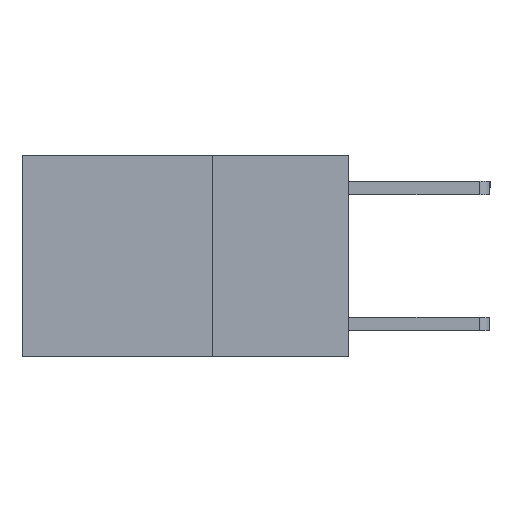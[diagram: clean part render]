
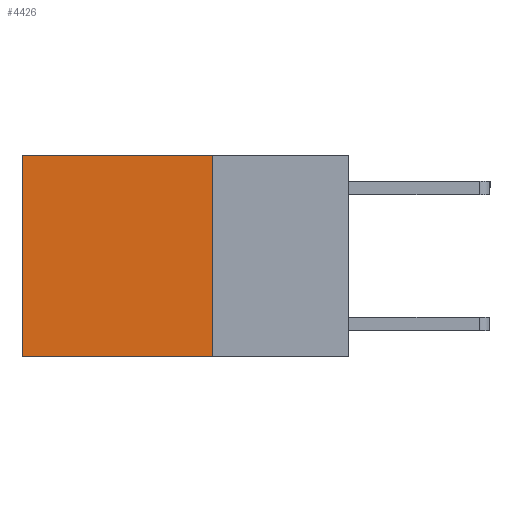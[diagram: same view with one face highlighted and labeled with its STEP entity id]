
A CAD part, left-side view. The second image highlights one B-rep face of the part: STEP entity #4426.
In plain terms, the highlighted planar face has unit normal (-1, 0, 0).
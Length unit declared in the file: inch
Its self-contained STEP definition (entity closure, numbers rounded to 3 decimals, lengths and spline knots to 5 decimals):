
#96 = EDGE_CURVE ( 'NONE', #2459, #6514, #1428, .T. ) ;
#484 = DIRECTION ( 'NONE',  ( 0., 1., 0. ) ) ;
#525 = DIRECTION ( 'NONE',  ( 0., 1., 0. ) ) ;
#591 = CARTESIAN_POINT ( 'NONE',  ( 0.2625, 0.25, 0. ) ) ;
#830 = CARTESIAN_POINT ( 'NONE',  ( 0.2625, 0.6, 0. ) ) ;
#1220 = LINE ( 'NONE', #8848, #2858 ) ;
#1428 = LINE ( 'NONE', #8766, #1678 ) ;
#1554 = VERTEX_POINT ( 'NONE', #6920 ) ;
#1678 = VECTOR ( 'NONE', #484, 39.37008 ) ;
#1773 = EDGE_CURVE ( 'NONE', #2459, #1554, #2699, .T. ) ;
#1987 = PLANE ( 'NONE',  #2639 ) ;
#2238 = VECTOR ( 'NONE', #9204, 39.37008 ) ;
#2419 = LINE ( 'NONE', #830, #2238 ) ;
#2459 = VERTEX_POINT ( 'NONE', #5392 ) ;
#2639 = AXIS2_PLACEMENT_3D ( 'NONE', #591, #5716, #7133 ) ;
#2699 = LINE ( 'NONE', #6378, #6075 ) ;
#2725 = ORIENTED_EDGE ( 'NONE', *, *, #9723, .F. ) ;
#2858 = VECTOR ( 'NONE', #525, 39.37008 ) ;
#3515 = FACE_OUTER_BOUND ( 'NONE', #7522, .T. ) ;
#3534 = VERTEX_POINT ( 'NONE', #4832 ) ;
#4105 = ORIENTED_EDGE ( 'NONE', *, *, #96, .T. ) ;
#4426 = ADVANCED_FACE ( 'NONE', ( #3515 ), #1987, .F. ) ;
#4832 = CARTESIAN_POINT ( 'NONE',  ( 0.2625, 0.6, -0.37 ) ) ;
#5392 = CARTESIAN_POINT ( 'NONE',  ( 0.2625, 0.25, 0. ) ) ;
#5699 = DIRECTION ( 'NONE',  ( 0., 0., -1. ) ) ;
#5716 = DIRECTION ( 'NONE',  ( 1., 0., 0. ) ) ;
#6075 = VECTOR ( 'NONE', #5699, 39.37008 ) ;
#6378 = CARTESIAN_POINT ( 'NONE',  ( 0.2625, 0.25, 0. ) ) ;
#6514 = VERTEX_POINT ( 'NONE', #8707 ) ;
#6920 = CARTESIAN_POINT ( 'NONE',  ( 0.2625, 0.25, -0.37 ) ) ;
#7105 = ORIENTED_EDGE ( 'NONE', *, *, #7531, .T. ) ;
#7133 = DIRECTION ( 'NONE',  ( 0., 0., -1. ) ) ;
#7522 = EDGE_LOOP ( 'NONE', ( #7105, #2725, #9555, #4105 ) ) ;
#7531 = EDGE_CURVE ( 'NONE', #6514, #3534, #2419, .T. ) ;
#8707 = CARTESIAN_POINT ( 'NONE',  ( 0.2625, 0.6, 0. ) ) ;
#8766 = CARTESIAN_POINT ( 'NONE',  ( 0.2625, 0.25, 0. ) ) ;
#8848 = CARTESIAN_POINT ( 'NONE',  ( 0.2625, 0.25, -0.37 ) ) ;
#9204 = DIRECTION ( 'NONE',  ( 0., 0., -1. ) ) ;
#9555 = ORIENTED_EDGE ( 'NONE', *, *, #1773, .F. ) ;
#9723 = EDGE_CURVE ( 'NONE', #1554, #3534, #1220, .T. ) ;
